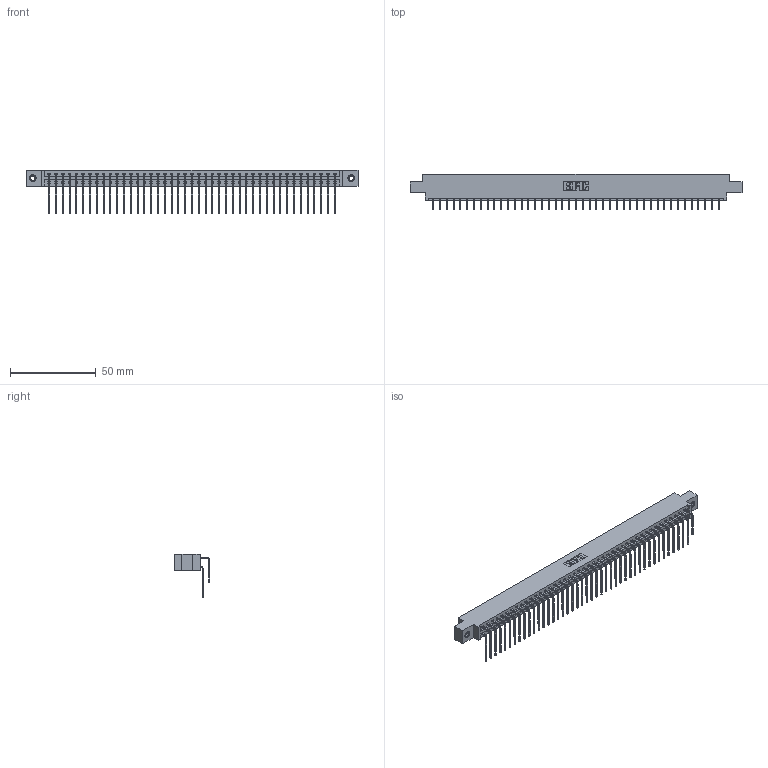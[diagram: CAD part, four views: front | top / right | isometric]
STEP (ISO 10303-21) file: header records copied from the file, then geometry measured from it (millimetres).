
FILE_DESCRIPTION (( 'STEP AP203' ), '1' );
FILE_NAME ('337-086-559-807.STEP', '2018-08-13T02:32:45', ( '' ), ( '' ), 'SwSTEP 2.0', 'SolidWorks 2016', '' );
FILE_SCHEMA (( 'CONFIG_CONTROL_DESIGN' ));
Length unit declared in the file: inch
Products named in the file (5): 345-292-001_559 Tail - 2; 345-250-001_345-250-005-103; 337-086-559-807; 337 Part_0.170 Offset - 0.156 Dia-TI; 345-292-001_558 559 Tail - 1
Assembly tree (89 placements, depth 2):
  337-086-559-807
    337 Part_0.170 Offset - 0.156 Dia-TI
    345-292-001_558 559 Tail - 1  x43
    345-292-001_559 Tail - 2  x43
    345-250-001_345-250-005-103  x2
Bounding box: 193.4 x 20.9 x 25.53 mm (x, y, z)
Volume: 20760 mm3; surface area: 26113.8 mm2
Topology: 89 solids, 89 shells, 4994 faces, 14821 edges, 9758 vertices
Faces by surface type: plane 3546, cylinder 1432, cone 12, torus 4
Entity records: 36312 total; most frequent: CARTESIAN_POINT 6144, ORIENTED_EDGE 6022, DIRECTION 5237, EDGE_CURVE 3011, VECTOR 2823, LINE 2823, VERTEX_POINT 2000, AXIS2_PLACEMENT_3D 1207
